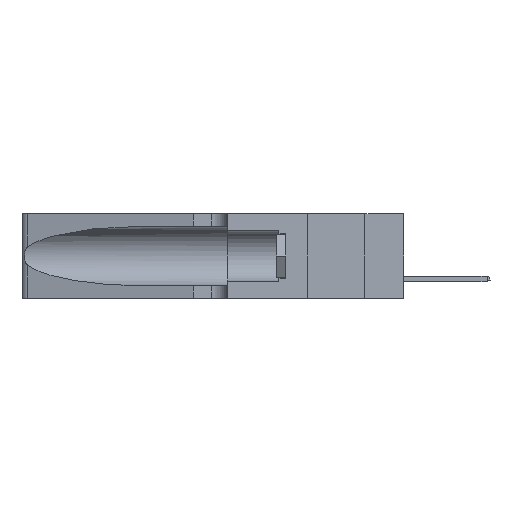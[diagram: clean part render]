
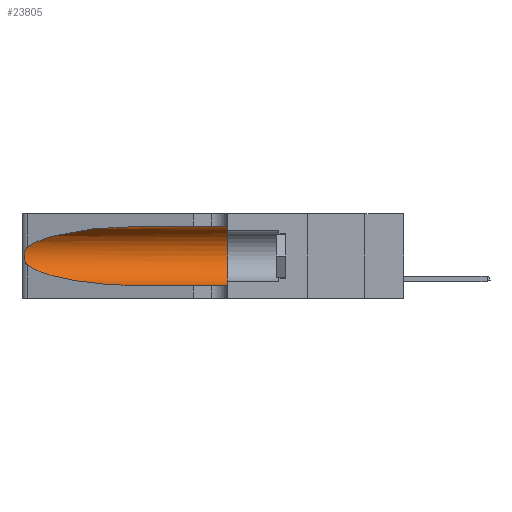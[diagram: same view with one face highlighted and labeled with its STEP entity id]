
A CAD part, left-side view. The second image highlights one B-rep face of the part: STEP entity #23805.
In plain terms, the highlighted cylindrical face has radius 3.308 mm (diameter 6.617 mm), a partial arc.
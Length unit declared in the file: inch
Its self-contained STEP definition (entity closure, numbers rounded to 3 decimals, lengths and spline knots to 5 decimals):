
#412 =( BOUNDED_CURVE ( )  B_SPLINE_CURVE ( 3, ( #24530, #10727, #18059, #29663 ),
 .UNSPECIFIED., .F., .T. ) 
 B_SPLINE_CURVE_WITH_KNOTS ( ( 4, 4 ),
 ( 3.44316, 4.71239 ),
 .UNSPECIFIED. ) 
 CURVE ( )  GEOMETRIC_REPRESENTATION_ITEM ( )  RATIONAL_B_SPLINE_CURVE ( ( 1., 0.87, 0.87, 1. ) ) 
 REPRESENTATION_ITEM ( '' )  );
#736 = CARTESIAN_POINT ( 'NONE',  ( 0.26075, 1.23896, 0.19203 ) ) ;
#1047 = CARTESIAN_POINT ( 'NONE',  ( 0.1305, 1.61858, 0.185 ) ) ;
#1292 = EDGE_CURVE ( 'NONE', #22967, #4225, #5653, .T. ) ;
#1605 = ORIENTED_EDGE ( 'NONE', *, *, #1292, .F. ) ;
#2259 = DIRECTION ( 'NONE',  ( 0., 0., -1. ) ) ;
#2988 = CARTESIAN_POINT ( 'NONE',  ( 0.25487, 1.22718, 0.14631 ) ) ;
#3169 = ORIENTED_EDGE ( 'NONE', *, *, #18479, .T. ) ;
#4225 = VERTEX_POINT ( 'NONE', #6084 ) ;
#4916 = EDGE_CURVE ( 'NONE', #16334, #9575, #28488, .T. ) ;
#5144 = DIRECTION ( 'NONE',  ( 0., -1., 0. ) ) ;
#5603 = CARTESIAN_POINT ( 'NONE',  ( 0.25856, 1.23593, 0.16098 ) ) ;
#5653 = LINE ( 'NONE', #19040, #29694 ) ;
#5812 = CARTESIAN_POINT ( 'NONE',  ( 0.25789, 1.23486, 0.15765 ) ) ;
#6084 = CARTESIAN_POINT ( 'NONE',  ( 0.1305, 0.35, 0.31525 ) ) ;
#6224 = EDGE_CURVE ( 'NONE', #4225, #20747, #13309, .T. ) ;
#6783 = CARTESIAN_POINT ( 'NONE',  ( 0.18966, 0.96281, 0.31525 ) ) ;
#6954 = CARTESIAN_POINT ( 'NONE',  ( 0.1305, 1.61858, 0.05475 ) ) ;
#8016 = CARTESIAN_POINT ( 'NONE',  ( 0.25487, 1.22718, 0.14631 ) ) ;
#9189 = CARTESIAN_POINT ( 'NONE',  ( 0.1305, 0.72297, 0.31525 ) ) ;
#9575 = VERTEX_POINT ( 'NONE', #8016 ) ;
#10177 = CARTESIAN_POINT ( 'NONE',  ( 0.25487, 1.22718, 0.22369 ) ) ;
#10727 = CARTESIAN_POINT ( 'NONE',  ( 0.2373, 1.15595, 0.08982 ) ) ;
#10861 = CARTESIAN_POINT ( 'NONE',  ( 0.1305, 0.35, 0.185 ) ) ;
#11234 = FACE_OUTER_BOUND ( 'NONE', #22442, .T. ) ;
#11722 = DIRECTION ( 'NONE',  ( 0., -1., 0. ) ) ;
#11754 = CARTESIAN_POINT ( 'NONE',  ( 0.2373, 1.15595, 0.28018 ) ) ;
#12261 =( BOUNDED_CURVE ( )  B_SPLINE_CURVE ( 3, ( #24935, #6783, #11754, #17533 ),
 .UNSPECIFIED., .F., .F. ) 
 B_SPLINE_CURVE_WITH_KNOTS ( ( 4, 4 ),
 ( 1.5708, 2.84003 ),
 .UNSPECIFIED. ) 
 CURVE ( )  GEOMETRIC_REPRESENTATION_ITEM ( )  RATIONAL_B_SPLINE_CURVE ( ( 1., 0.87, 0.87, 1. ) ) 
 REPRESENTATION_ITEM ( '' )  );
#12661 = CARTESIAN_POINT ( 'NONE',  ( 0.25487, 1.22718, 0.22369 ) ) ;
#12732 = LINE ( 'NONE', #6954, #19222 ) ;
#12733 = CARTESIAN_POINT ( 'NONE',  ( 0.26018, 1.23835, 0.19895 ) ) ;
#12815 = EDGE_CURVE ( 'NONE', #9575, #28446, #412, .T. ) ;
#12842 = CARTESIAN_POINT ( 'NONE',  ( 0.25787, 1.23484, 0.2124 ) ) ;
#12866 = ORIENTED_EDGE ( 'NONE', *, *, #12815, .T. ) ;
#13309 = CIRCLE ( 'NONE', #28558, 0.13025 ) ;
#13455 = ORIENTED_EDGE ( 'NONE', *, *, #16574, .T. ) ;
#16334 = VERTEX_POINT ( 'NONE', #12661 ) ;
#16574 = EDGE_CURVE ( 'NONE', #22967, #16334, #12261, .T. ) ;
#17096 = CARTESIAN_POINT ( 'NONE',  ( 0.25639, 1.23186, 0.15144 ) ) ;
#17533 = CARTESIAN_POINT ( 'NONE',  ( 0.25487, 1.22718, 0.22369 ) ) ;
#17664 = CARTESIAN_POINT ( 'NONE',  ( 0.1305, 0.72297, 0.05475 ) ) ;
#18059 = CARTESIAN_POINT ( 'NONE',  ( 0.18966, 0.96281, 0.05475 ) ) ;
#18479 = EDGE_CURVE ( 'NONE', #28446, #20747, #12732, .T. ) ;
#19040 = CARTESIAN_POINT ( 'NONE',  ( 0.1305, 1.61858, 0.31525 ) ) ;
#19083 = AXIS2_PLACEMENT_3D ( 'NONE', #1047, #11722, #2259 ) ;
#19222 = VECTOR ( 'NONE', #28594, 39.37008 ) ;
#19415 = ORIENTED_EDGE ( 'NONE', *, *, #4916, .T. ) ;
#20002 = ORIENTED_EDGE ( 'NONE', *, *, #6224, .F. ) ;
#20747 = VERTEX_POINT ( 'NONE', #25095 ) ;
#21717 = CARTESIAN_POINT ( 'NONE',  ( 0.26075, 1.23896, 0.178 ) ) ;
#22046 = CARTESIAN_POINT ( 'NONE',  ( 0.25555, 1.22994, 0.2215 ) ) ;
#22114 = DIRECTION ( 'NONE',  ( 0., 1., 0. ) ) ;
#22442 = EDGE_LOOP ( 'NONE', ( #13455, #19415, #12866, #3169, #20002, #1605 ) ) ;
#22967 = VERTEX_POINT ( 'NONE', #9189 ) ;
#23805 = ADVANCED_FACE ( 'NONE', ( #11234 ), #25008, .F. ) ;
#24273 = CARTESIAN_POINT ( 'NONE',  ( 0.26017, 1.23833, 0.17102 ) ) ;
#24530 = CARTESIAN_POINT ( 'NONE',  ( 0.25487, 1.22718, 0.14631 ) ) ;
#24935 = CARTESIAN_POINT ( 'NONE',  ( 0.1305, 0.72297, 0.31525 ) ) ;
#25008 = CYLINDRICAL_SURFACE ( 'NONE', #19083, 0.13025 ) ;
#25095 = CARTESIAN_POINT ( 'NONE',  ( 0.1305, 0.35, 0.05475 ) ) ;
#26522 = CARTESIAN_POINT ( 'NONE',  ( 0.25555, 1.22993, 0.14849 ) ) ;
#26725 = CARTESIAN_POINT ( 'NONE',  ( 0.25639, 1.23184, 0.21858 ) ) ;
#28446 = VERTEX_POINT ( 'NONE', #17664 ) ;
#28488 = B_SPLINE_CURVE_WITH_KNOTS ( 'NONE', 3,
 ( #10177, #22046, #26725, #12842, #29094, #12733, #736, #21717, #24273, #5603, #5812, #17096, #26522, #2988 ),
 .UNSPECIFIED., .F., .F.,
 ( 4, 2, 2, 2, 2, 2, 4 ),
 ( 0., 0.00027, 0.00053, 0.00107, 0.0016, 0.00187, 0.00214 ),
 .UNSPECIFIED. ) ;
#28558 = AXIS2_PLACEMENT_3D ( 'NONE', #10861, #22114, #29264 ) ;
#28594 = DIRECTION ( 'NONE',  ( 0., -1., 0. ) ) ;
#29094 = CARTESIAN_POINT ( 'NONE',  ( 0.25854, 1.2359, 0.20912 ) ) ;
#29264 = DIRECTION ( 'NONE',  ( 0., 0., 1. ) ) ;
#29663 = CARTESIAN_POINT ( 'NONE',  ( 0.1305, 0.72297, 0.05475 ) ) ;
#29694 = VECTOR ( 'NONE', #5144, 39.37008 ) ;
